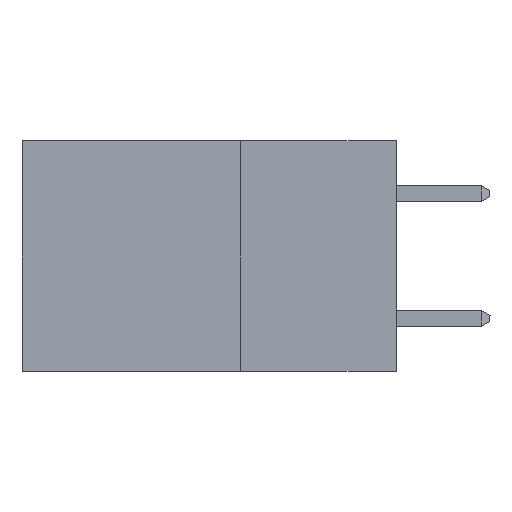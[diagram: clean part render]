
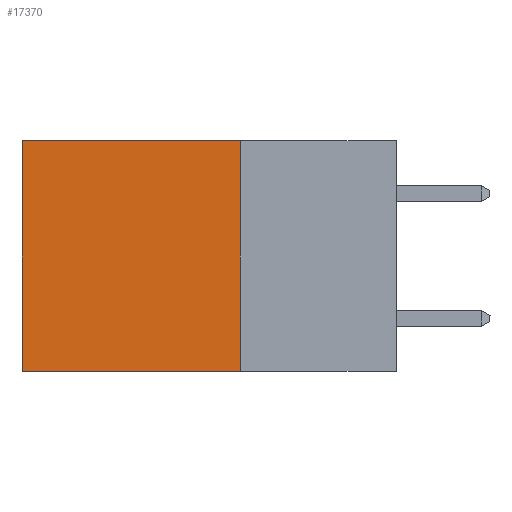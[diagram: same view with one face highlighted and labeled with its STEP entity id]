
A CAD part, left-side view. The second image highlights one B-rep face of the part: STEP entity #17370.
In plain terms, the highlighted planar face has unit normal (-1, 0, 0).
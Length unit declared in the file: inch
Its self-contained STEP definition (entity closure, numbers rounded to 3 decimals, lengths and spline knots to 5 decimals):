
#707 = VECTOR ( 'NONE', #9359, 39.37008 ) ;
#745 = VECTOR ( 'NONE', #4880, 39.37008 ) ;
#2254 = ORIENTED_EDGE ( 'NONE', *, *, #17061, .T. ) ;
#3159 = CARTESIAN_POINT ( 'NONE',  ( 0.2615, 0.25, 0. ) ) ;
#3574 = CARTESIAN_POINT ( 'NONE',  ( 0.2615, 0.6, 0. ) ) ;
#3986 = CARTESIAN_POINT ( 'NONE',  ( 0.2615, 0.6, -0.37 ) ) ;
#4047 = ORIENTED_EDGE ( 'NONE', *, *, #7159, .F. ) ;
#4750 = AXIS2_PLACEMENT_3D ( 'NONE', #6771, #8713, #22229 ) ;
#4838 = PLANE ( 'NONE',  #4750 ) ;
#4848 = LINE ( 'NONE', #3986, #19121 ) ;
#4880 = DIRECTION ( 'NONE',  ( 0., 0., -1. ) ) ;
#5192 = EDGE_LOOP ( 'NONE', ( #2254, #4047, #6569, #16351 ) ) ;
#5791 = VERTEX_POINT ( 'NONE', #3574 ) ;
#6569 = ORIENTED_EDGE ( 'NONE', *, *, #11831, .F. ) ;
#6771 = CARTESIAN_POINT ( 'NONE',  ( 0.2615, 0.25, -0.37 ) ) ;
#7159 = EDGE_CURVE ( 'NONE', #11695, #21766, #9802, .T. ) ;
#7827 = FACE_OUTER_BOUND ( 'NONE', #5192, .T. ) ;
#8155 = EDGE_CURVE ( 'NONE', #16752, #5791, #8885, .T. ) ;
#8713 = DIRECTION ( 'NONE',  ( 1., 0., 0. ) ) ;
#8885 = LINE ( 'NONE', #23657, #18026 ) ;
#9359 = DIRECTION ( 'NONE',  ( 0., 1., 0. ) ) ;
#9802 = LINE ( 'NONE', #20964, #707 ) ;
#11695 = VERTEX_POINT ( 'NONE', #12478 ) ;
#11831 = EDGE_CURVE ( 'NONE', #16752, #11695, #15641, .T. ) ;
#12478 = CARTESIAN_POINT ( 'NONE',  ( 0.2615, 0.25, -0.37 ) ) ;
#13748 = CARTESIAN_POINT ( 'NONE',  ( 0.2615, 0.6, -0.37 ) ) ;
#14548 = CARTESIAN_POINT ( 'NONE',  ( 0.2615, 0.25, -0.37 ) ) ;
#15641 = LINE ( 'NONE', #14548, #745 ) ;
#16043 = DIRECTION ( 'NONE',  ( 0., 1., 0. ) ) ;
#16351 = ORIENTED_EDGE ( 'NONE', *, *, #8155, .T. ) ;
#16752 = VERTEX_POINT ( 'NONE', #3159 ) ;
#17061 = EDGE_CURVE ( 'NONE', #5791, #21766, #4848, .T. ) ;
#17370 = ADVANCED_FACE ( 'NONE', ( #7827 ), #4838, .F. ) ;
#18026 = VECTOR ( 'NONE', #16043, 39.37008 ) ;
#19121 = VECTOR ( 'NONE', #19528, 39.37008 ) ;
#19528 = DIRECTION ( 'NONE',  ( 0., 0., -1. ) ) ;
#20964 = CARTESIAN_POINT ( 'NONE',  ( 0.2615, 0.25, -0.37 ) ) ;
#21766 = VERTEX_POINT ( 'NONE', #13748 ) ;
#22229 = DIRECTION ( 'NONE',  ( 0., 0., -1. ) ) ;
#23657 = CARTESIAN_POINT ( 'NONE',  ( 0.2615, 0.25, 0. ) ) ;
